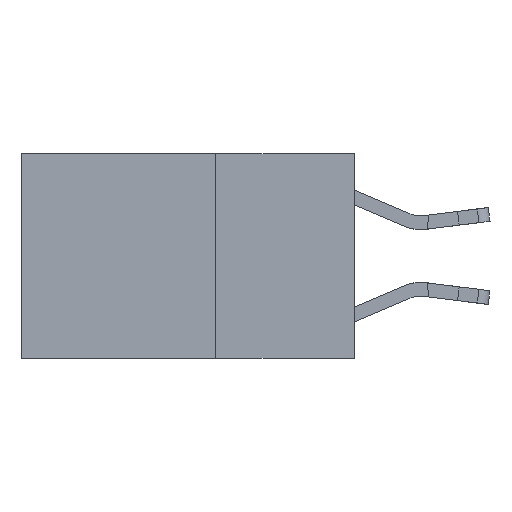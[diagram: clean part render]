
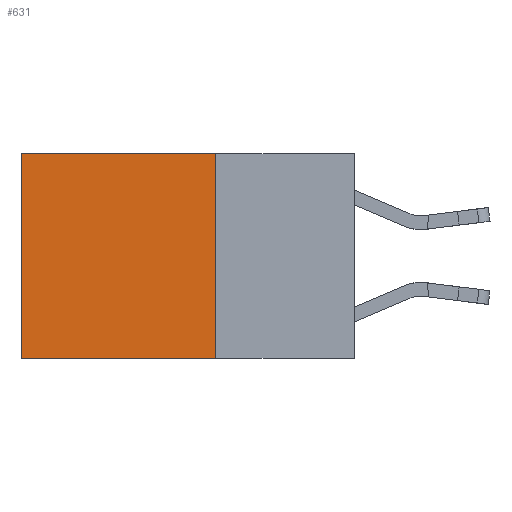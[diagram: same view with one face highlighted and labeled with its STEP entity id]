
A CAD part, left-side view. The second image highlights one B-rep face of the part: STEP entity #631.
In plain terms, the highlighted planar face has unit normal (-1, 0, 0).
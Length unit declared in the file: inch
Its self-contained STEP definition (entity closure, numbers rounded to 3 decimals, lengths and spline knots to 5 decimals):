
#445 = DIRECTION ( 'NONE',  ( 1., 0., 0. ) ) ;
#631 = ADVANCED_FACE ( 'NONE', ( #12881 ), #7862, .F. ) ;
#1283 = VERTEX_POINT ( 'NONE', #4043 ) ;
#1355 = LINE ( 'NONE', #5789, #13756 ) ;
#1924 = VECTOR ( 'NONE', #2077, 39.37008 ) ;
#2077 = DIRECTION ( 'NONE',  ( 0., 0., -1. ) ) ;
#2333 = LINE ( 'NONE', #10621, #1924 ) ;
#3577 = ORIENTED_EDGE ( 'NONE', *, *, #9383, .T. ) ;
#4043 = CARTESIAN_POINT ( 'NONE',  ( 0.2625, 0.6, -0.37 ) ) ;
#4344 = EDGE_CURVE ( 'NONE', #14800, #14907, #7979, .T. ) ;
#4358 = ORIENTED_EDGE ( 'NONE', *, *, #12542, .F. ) ;
#4605 = DIRECTION ( 'NONE',  ( 0., 0., -1. ) ) ;
#4841 = CARTESIAN_POINT ( 'NONE',  ( 0.2625, 0.25, -0.37 ) ) ;
#5707 = AXIS2_PLACEMENT_3D ( 'NONE', #13668, #445, #9085 ) ;
#5789 = CARTESIAN_POINT ( 'NONE',  ( 0.2625, 0.25, 0. ) ) ;
#6069 = VECTOR ( 'NONE', #14707, 39.37008 ) ;
#6451 = LINE ( 'NONE', #6504, #6069 ) ;
#6504 = CARTESIAN_POINT ( 'NONE',  ( 0.2625, 0.25, -0.37 ) ) ;
#7592 = VECTOR ( 'NONE', #8927, 39.37008 ) ;
#7862 = PLANE ( 'NONE',  #5707 ) ;
#7979 = LINE ( 'NONE', #10133, #7592 ) ;
#8492 = ORIENTED_EDGE ( 'NONE', *, *, #8788, .F. ) ;
#8788 = EDGE_CURVE ( 'NONE', #14800, #10032, #1355, .T. ) ;
#8927 = DIRECTION ( 'NONE',  ( 0., 1., 0. ) ) ;
#9085 = DIRECTION ( 'NONE',  ( 0., 0., -1. ) ) ;
#9383 = EDGE_CURVE ( 'NONE', #14907, #1283, #2333, .T. ) ;
#9732 = CARTESIAN_POINT ( 'NONE',  ( 0.2625, 0.25, 0. ) ) ;
#10032 = VERTEX_POINT ( 'NONE', #4841 ) ;
#10133 = CARTESIAN_POINT ( 'NONE',  ( 0.2625, 0.25, 0. ) ) ;
#10621 = CARTESIAN_POINT ( 'NONE',  ( 0.2625, 0.6, 0. ) ) ;
#10995 = CARTESIAN_POINT ( 'NONE',  ( 0.2625, 0.6, 0. ) ) ;
#12469 = ORIENTED_EDGE ( 'NONE', *, *, #4344, .T. ) ;
#12542 = EDGE_CURVE ( 'NONE', #10032, #1283, #6451, .T. ) ;
#12881 = FACE_OUTER_BOUND ( 'NONE', #13015, .T. ) ;
#13015 = EDGE_LOOP ( 'NONE', ( #3577, #4358, #8492, #12469 ) ) ;
#13668 = CARTESIAN_POINT ( 'NONE',  ( 0.2625, 0.25, 0. ) ) ;
#13756 = VECTOR ( 'NONE', #4605, 39.37008 ) ;
#14707 = DIRECTION ( 'NONE',  ( 0., 1., 0. ) ) ;
#14800 = VERTEX_POINT ( 'NONE', #9732 ) ;
#14907 = VERTEX_POINT ( 'NONE', #10995 ) ;
